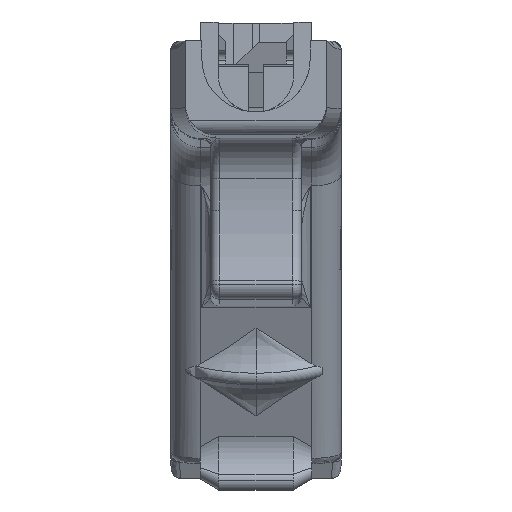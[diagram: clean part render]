
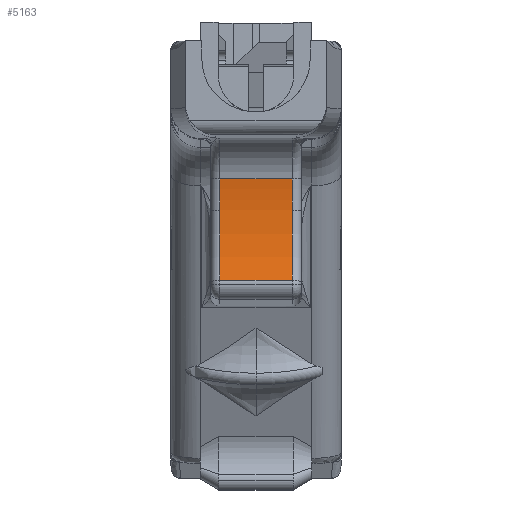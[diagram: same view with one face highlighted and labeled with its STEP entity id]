
A CAD part, top view. The second image highlights one B-rep face of the part: STEP entity #5163.
In plain terms, the highlighted cylindrical face has radius 41.155 mm (diameter 82.31 mm), a partial arc.
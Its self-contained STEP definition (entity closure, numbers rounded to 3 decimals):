
#110 = DIRECTION ( 'NONE',  ( 1., 0., 0. ) ) ;
#229 = CIRCLE ( 'NONE', #12835, 41.155 ) ;
#613 = CARTESIAN_POINT ( 'NONE',  ( -6.223, -29.007, 0.864 ) ) ;
#1020 = EDGE_CURVE ( 'NONE', #4812, #5971, #7143, .T. ) ;
#1030 = VERTEX_POINT ( 'NONE', #1586 ) ;
#1160 = DIRECTION ( 'NONE',  ( -1., 0., 0. ) ) ;
#1586 = CARTESIAN_POINT ( 'NONE',  ( -6.223, -29.007, -40.291 ) ) ;
#1632 = DIRECTION ( 'NONE',  ( 0., 0., -1. ) ) ;
#2009 = VECTOR ( 'NONE', #10383, 1000. ) ;
#2057 = EDGE_CURVE ( 'NONE', #4812, #10628, #229, .T. ) ;
#2248 = DIRECTION ( 'NONE',  ( 0., 0., 1. ) ) ;
#2522 = AXIS2_PLACEMENT_3D ( 'NONE', #6263, #110, #7259 ) ;
#2593 = AXIS2_PLACEMENT_3D ( 'NONE', #613, #7771, #1632 ) ;
#3045 = DIRECTION ( 'NONE',  ( -1., 0., 0. ) ) ;
#3341 = CYLINDRICAL_SURFACE ( 'NONE', #4052, 41.155 ) ;
#3561 = CARTESIAN_POINT ( 'NONE',  ( 6.223, -29.007, 0.864 ) ) ;
#3819 = CARTESIAN_POINT ( 'NONE',  ( 6.223, -40.969, -38.514 ) ) ;
#3981 = CIRCLE ( 'NONE', #2593, 41.155 ) ;
#4052 = AXIS2_PLACEMENT_3D ( 'NONE', #7345, #1160, #2248 ) ;
#4423 = VERTEX_POINT ( 'NONE', #11586 ) ;
#4596 = DIRECTION ( 'NONE',  ( 0., 0., -1. ) ) ;
#4714 = CARTESIAN_POINT ( 'NONE',  ( 6.223, -29.007, -40.291 ) ) ;
#4812 = VERTEX_POINT ( 'NONE', #3819 ) ;
#4998 = ORIENTED_EDGE ( 'NONE', *, *, #5959, .T. ) ;
#5163 = ADVANCED_FACE ( 'NONE', ( #8760 ), #3341, .F. ) ;
#5717 = CIRCLE ( 'NONE', #9997, 41.155 ) ;
#5959 = EDGE_CURVE ( 'NONE', #10999, #4423, #12989, .T. ) ;
#5971 = VERTEX_POINT ( 'NONE', #12287 ) ;
#6263 = CARTESIAN_POINT ( 'NONE',  ( 6.223, -29.007, 0.864 ) ) ;
#6406 = ORIENTED_EDGE ( 'NONE', *, *, #7283, .T. ) ;
#7133 = DIRECTION ( 'NONE',  ( -1., 0., 0. ) ) ;
#7143 = LINE ( 'NONE', #11342, #2009 ) ;
#7259 = DIRECTION ( 'NONE',  ( 0., 0., -1. ) ) ;
#7283 = EDGE_CURVE ( 'NONE', #4423, #1030, #3981, .T. ) ;
#7345 = CARTESIAN_POINT ( 'NONE',  ( 7.747, -29.007, 0.864 ) ) ;
#7771 = DIRECTION ( 'NONE',  ( -1., 0., 0. ) ) ;
#8063 = EDGE_CURVE ( 'NONE', #10628, #10999, #9530, .T. ) ;
#8384 = EDGE_CURVE ( 'NONE', #1030, #5971, #5717, .T. ) ;
#8467 = CARTESIAN_POINT ( 'NONE',  ( 6.223, -23.613, -39.936 ) ) ;
#8694 = ORIENTED_EDGE ( 'NONE', *, *, #8384, .T. ) ;
#8760 = FACE_OUTER_BOUND ( 'NONE', #9183, .T. ) ;
#9130 = CARTESIAN_POINT ( 'NONE',  ( 7.747, -23.613, -39.936 ) ) ;
#9156 = CARTESIAN_POINT ( 'NONE',  ( -6.223, -29.007, 0.864 ) ) ;
#9183 = EDGE_LOOP ( 'NONE', ( #4998, #6406, #8694, #9964, #11558, #13114 ) ) ;
#9530 = CIRCLE ( 'NONE', #2522, 41.155 ) ;
#9964 = ORIENTED_EDGE ( 'NONE', *, *, #1020, .F. ) ;
#9997 = AXIS2_PLACEMENT_3D ( 'NONE', #9156, #3045, #10213 ) ;
#10213 = DIRECTION ( 'NONE',  ( 0., 0., -1. ) ) ;
#10222 = VECTOR ( 'NONE', #7133, 1000. ) ;
#10383 = DIRECTION ( 'NONE',  ( -1., 0., 0. ) ) ;
#10628 = VERTEX_POINT ( 'NONE', #4714 ) ;
#10714 = DIRECTION ( 'NONE',  ( 1., 0., 0. ) ) ;
#10999 = VERTEX_POINT ( 'NONE', #8467 ) ;
#11342 = CARTESIAN_POINT ( 'NONE',  ( 7.747, -40.969, -38.514 ) ) ;
#11558 = ORIENTED_EDGE ( 'NONE', *, *, #2057, .T. ) ;
#11586 = CARTESIAN_POINT ( 'NONE',  ( -6.223, -23.613, -39.936 ) ) ;
#12287 = CARTESIAN_POINT ( 'NONE',  ( -6.223, -40.969, -38.514 ) ) ;
#12835 = AXIS2_PLACEMENT_3D ( 'NONE', #3561, #10714, #4596 ) ;
#12989 = LINE ( 'NONE', #9130, #10222 ) ;
#13114 = ORIENTED_EDGE ( 'NONE', *, *, #8063, .T. ) ;
